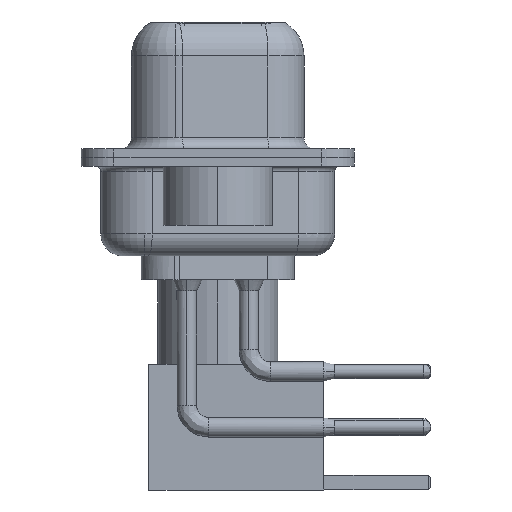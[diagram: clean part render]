
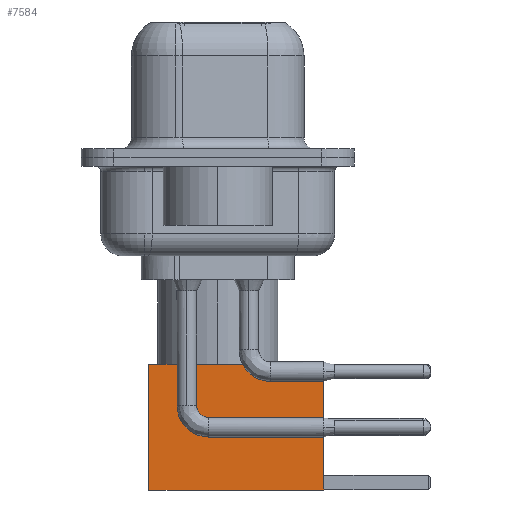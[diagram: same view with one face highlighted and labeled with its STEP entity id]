
A CAD part, left-side view. The second image highlights one B-rep face of the part: STEP entity #7584.
In plain terms, the highlighted face is planar.
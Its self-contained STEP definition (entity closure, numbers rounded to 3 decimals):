
#368 = DIRECTION ( 'NONE',  ( -1., 0., 0. ) ) ;
#585 = VERTEX_POINT ( 'NONE', #9106 ) ;
#1640 = DIRECTION ( 'NONE',  ( 0., 0., 1. ) ) ;
#3853 = ORIENTED_EDGE ( 'NONE', *, *, #18713, .F. ) ;
#4160 = CARTESIAN_POINT ( 'NONE',  ( -2.875, 2.875, 0. ) ) ;
#4639 = EDGE_LOOP ( 'NONE', ( #10328, #5860, #9161, #3853 ) ) ;
#4722 = CARTESIAN_POINT ( 'NONE',  ( 0., 2.875, 0. ) ) ;
#5012 = CARTESIAN_POINT ( 'NONE',  ( -2.875, 2.875, 0. ) ) ;
#5449 = EDGE_CURVE ( 'NONE', #17436, #11049, #14147, .T. ) ;
#5860 = ORIENTED_EDGE ( 'NONE', *, *, #13633, .T. ) ;
#6524 = LINE ( 'NONE', #13580, #13698 ) ;
#6879 = AXIS2_PLACEMENT_3D ( 'NONE', #14675, #14869, #1640 ) ;
#7386 = VECTOR ( 'NONE', #14581, 1000. ) ;
#7509 = FACE_OUTER_BOUND ( 'NONE', #4639, .T. ) ;
#7584 = ADVANCED_FACE ( 'NONE', ( #7509 ), #13297, .T. ) ;
#7956 = DIRECTION ( 'NONE',  ( 0., 0., -1. ) ) ;
#8408 = CARTESIAN_POINT ( 'NONE',  ( 2.875, 2.875, 0. ) ) ;
#9106 = CARTESIAN_POINT ( 'NONE',  ( 2.875, 2.875, 0. ) ) ;
#9161 = ORIENTED_EDGE ( 'NONE', *, *, #5449, .F. ) ;
#9322 = DIRECTION ( 'NONE',  ( -1., 0., 0. ) ) ;
#9821 = CARTESIAN_POINT ( 'NONE',  ( 2.875, 2.875, 8. ) ) ;
#10328 = ORIENTED_EDGE ( 'NONE', *, *, #15005, .T. ) ;
#11049 = VERTEX_POINT ( 'NONE', #4160 ) ;
#13297 = PLANE ( 'NONE',  #6879 ) ;
#13580 = CARTESIAN_POINT ( 'NONE',  ( 0., 2.875, 8. ) ) ;
#13633 = EDGE_CURVE ( 'NONE', #585, #11049, #16611, .T. ) ;
#13698 = VECTOR ( 'NONE', #368, 1000. ) ;
#14147 = LINE ( 'NONE', #5012, #15790 ) ;
#14581 = DIRECTION ( 'NONE',  ( 0., 0., -1. ) ) ;
#14675 = CARTESIAN_POINT ( 'NONE',  ( 2.875, 2.875, 0. ) ) ;
#14826 = CARTESIAN_POINT ( 'NONE',  ( -2.875, 2.875, 8. ) ) ;
#14869 = DIRECTION ( 'NONE',  ( 0., 1., 0. ) ) ;
#15005 = EDGE_CURVE ( 'NONE', #17190, #585, #17354, .T. ) ;
#15790 = VECTOR ( 'NONE', #7956, 1000. ) ;
#16611 = LINE ( 'NONE', #4722, #18339 ) ;
#17190 = VERTEX_POINT ( 'NONE', #9821 ) ;
#17354 = LINE ( 'NONE', #8408, #7386 ) ;
#17436 = VERTEX_POINT ( 'NONE', #14826 ) ;
#18339 = VECTOR ( 'NONE', #9322, 1000. ) ;
#18713 = EDGE_CURVE ( 'NONE', #17190, #17436, #6524, .T. ) ;
